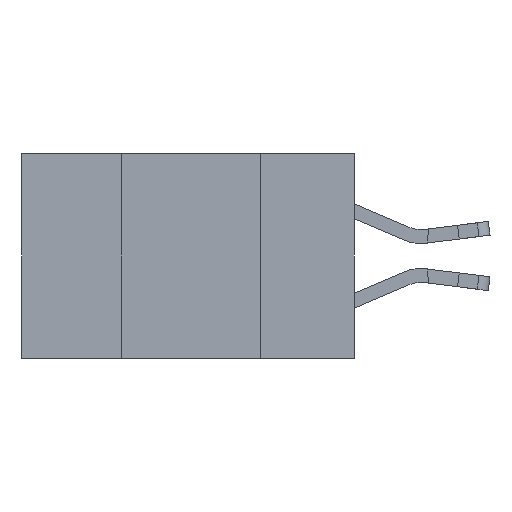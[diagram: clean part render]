
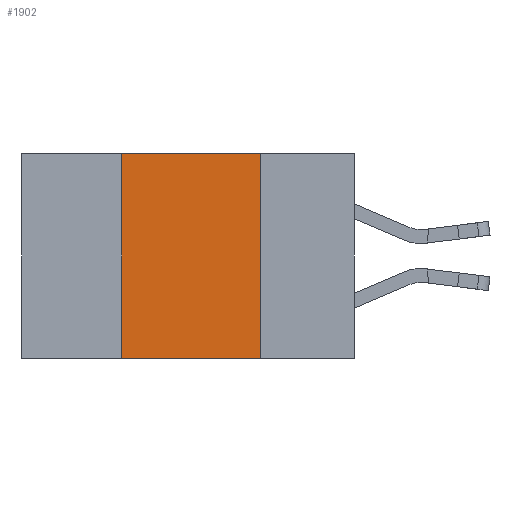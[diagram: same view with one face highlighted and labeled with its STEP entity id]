
A CAD part, left-side view. The second image highlights one B-rep face of the part: STEP entity #1902.
In plain terms, the highlighted planar face has unit normal (-1, 0, 0).
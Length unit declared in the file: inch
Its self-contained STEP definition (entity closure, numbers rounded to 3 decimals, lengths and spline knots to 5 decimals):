
#193 = EDGE_LOOP ( 'NONE', ( #2734, #3059, #3074, #2782 ) ) ;
#338 = CARTESIAN_POINT ( 'NONE',  ( 0., 0.17, 0. ) ) ;
#645 = CARTESIAN_POINT ( 'NONE',  ( 0., 0.42, -0.37 ) ) ;
#1175 = LINE ( 'NONE', #5342, #3744 ) ;
#1607 = LINE ( 'NONE', #10950, #10920 ) ;
#1871 = PLANE ( 'NONE',  #7533 ) ;
#1902 = ADVANCED_FACE ( 'NONE', ( #4911 ), #1871, .F. ) ;
#2075 = CARTESIAN_POINT ( 'NONE',  ( 0., 0.6, 0. ) ) ;
#2705 = VERTEX_POINT ( 'NONE', #338 ) ;
#2734 = ORIENTED_EDGE ( 'NONE', *, *, #7103, .F. ) ;
#2782 = ORIENTED_EDGE ( 'NONE', *, *, #4645, .T. ) ;
#2945 = DIRECTION ( 'NONE',  ( 0., -1., 0. ) ) ;
#3059 = ORIENTED_EDGE ( 'NONE', *, *, #5871, .F. ) ;
#3074 = ORIENTED_EDGE ( 'NONE', *, *, #5854, .F. ) ;
#3230 = VERTEX_POINT ( 'NONE', #5073 ) ;
#3710 = DIRECTION ( 'NONE',  ( 0., 0., 1. ) ) ;
#3744 = VECTOR ( 'NONE', #7215, 39.37008 ) ;
#3930 = VECTOR ( 'NONE', #3710, 39.37008 ) ;
#4633 = CARTESIAN_POINT ( 'NONE',  ( 0., 0.42, 0. ) ) ;
#4645 = EDGE_CURVE ( 'NONE', #10278, #7122, #1607, .T. ) ;
#4911 = FACE_OUTER_BOUND ( 'NONE', #193, .T. ) ;
#5073 = CARTESIAN_POINT ( 'NONE',  ( 0., 0.42, 0. ) ) ;
#5342 = CARTESIAN_POINT ( 'NONE',  ( 0., 0.17, 0. ) ) ;
#5378 = CARTESIAN_POINT ( 'NONE',  ( 0., 0.17, -0.37 ) ) ;
#5573 = DIRECTION ( 'NONE',  ( 0., -1., 0. ) ) ;
#5814 = DIRECTION ( 'NONE',  ( 0., 0., -1. ) ) ;
#5854 = EDGE_CURVE ( 'NONE', #10278, #3230, #8676, .T. ) ;
#5871 = EDGE_CURVE ( 'NONE', #3230, #2705, #8150, .T. ) ;
#7103 = EDGE_CURVE ( 'NONE', #2705, #7122, #1175, .T. ) ;
#7122 = VERTEX_POINT ( 'NONE', #5378 ) ;
#7215 = DIRECTION ( 'NONE',  ( 0., 0., -1. ) ) ;
#7533 = AXIS2_PLACEMENT_3D ( 'NONE', #2075, #10664, #5814 ) ;
#8150 = LINE ( 'NONE', #10848, #10708 ) ;
#8676 = LINE ( 'NONE', #4633, #3930 ) ;
#10278 = VERTEX_POINT ( 'NONE', #645 ) ;
#10664 = DIRECTION ( 'NONE',  ( 1., 0., 0. ) ) ;
#10708 = VECTOR ( 'NONE', #5573, 39.37008 ) ;
#10848 = CARTESIAN_POINT ( 'NONE',  ( 0., 0.6, 0. ) ) ;
#10920 = VECTOR ( 'NONE', #2945, 39.37008 ) ;
#10950 = CARTESIAN_POINT ( 'NONE',  ( 0., 0.6, -0.37 ) ) ;
